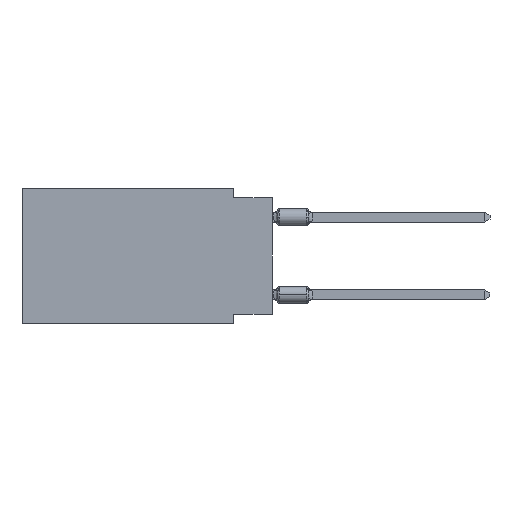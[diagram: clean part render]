
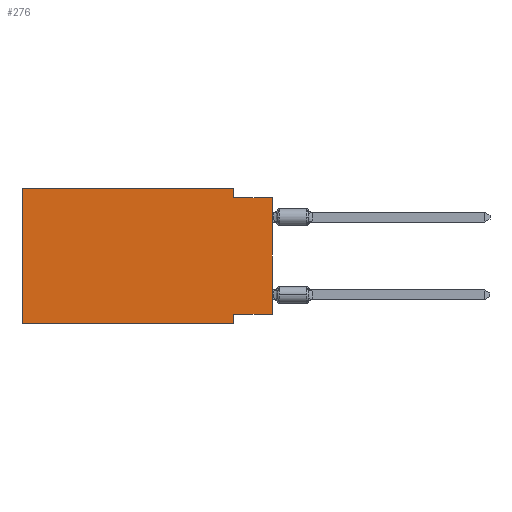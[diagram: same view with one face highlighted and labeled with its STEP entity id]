
A CAD part, left-side view. The second image highlights one B-rep face of the part: STEP entity #276.
In plain terms, the highlighted planar face has unit normal (-1, 0, 0).
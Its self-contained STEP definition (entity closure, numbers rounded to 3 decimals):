
#120 = LINE ( 'NONE', #13959, #4596 ) ;
#276 = ADVANCED_FACE ( 'NONE', ( #6881 ), #6651, .F. ) ;
#680 = DIRECTION ( 'NONE',  ( 0., 0., -1. ) ) ;
#1048 = VERTEX_POINT ( 'NONE', #13488 ) ;
#1146 = CARTESIAN_POINT ( 'NONE',  ( 0., 0., -8.255 ) ) ;
#1196 = VERTEX_POINT ( 'NONE', #15005 ) ;
#1869 = VECTOR ( 'NONE', #13306, 1000. ) ;
#1875 = VERTEX_POINT ( 'NONE', #13358 ) ;
#1990 = VECTOR ( 'NONE', #680, 1000. ) ;
#2413 = VECTOR ( 'NONE', #12455, 1000. ) ;
#2674 = VECTOR ( 'NONE', #12764, 1000. ) ;
#2703 = LINE ( 'NONE', #12063, #1869 ) ;
#2717 = ORIENTED_EDGE ( 'NONE', *, *, #8600, .T. ) ;
#2774 = CARTESIAN_POINT ( 'NONE',  ( 0., 0., 0. ) ) ;
#3293 = LINE ( 'NONE', #3523, #8495 ) ;
#3523 = CARTESIAN_POINT ( 'NONE',  ( 0., 0., -0.635 ) ) ;
#4596 = VECTOR ( 'NONE', #4800, 1000. ) ;
#4697 = CARTESIAN_POINT ( 'NONE',  ( 0., 2.54, -8.255 ) ) ;
#4733 = VECTOR ( 'NONE', #13228, 1000. ) ;
#4800 = DIRECTION ( 'NONE',  ( 0., -1., 0. ) ) ;
#5105 = CARTESIAN_POINT ( 'NONE',  ( 0., 0., -0.635 ) ) ;
#5641 = ORIENTED_EDGE ( 'NONE', *, *, #11929, .F. ) ;
#6446 = VERTEX_POINT ( 'NONE', #13236 ) ;
#6459 = VECTOR ( 'NONE', #9847, 1000. ) ;
#6506 = LINE ( 'NONE', #11202, #1990 ) ;
#6651 = PLANE ( 'NONE',  #11452 ) ;
#6821 = LINE ( 'NONE', #1146, #2674 ) ;
#6881 = FACE_OUTER_BOUND ( 'NONE', #9956, .T. ) ;
#7148 = ORIENTED_EDGE ( 'NONE', *, *, #14521, .F. ) ;
#7232 = CARTESIAN_POINT ( 'NONE',  ( 0., 16.383, -8.89 ) ) ;
#7884 = VERTEX_POINT ( 'NONE', #5105 ) ;
#8495 = VECTOR ( 'NONE', #12664, 1000. ) ;
#8591 = VERTEX_POINT ( 'NONE', #4697 ) ;
#8600 = EDGE_CURVE ( 'NONE', #12624, #7884, #9380, .T. ) ;
#9380 = LINE ( 'NONE', #2774, #4733 ) ;
#9426 = EDGE_CURVE ( 'NONE', #1875, #1048, #10852, .T. ) ;
#9847 = DIRECTION ( 'NONE',  ( 0., -1., 0. ) ) ;
#9956 = EDGE_LOOP ( 'NONE', ( #2717, #11241, #13002, #7148, #12438, #12199, #5641, #10058 ) ) ;
#10058 = ORIENTED_EDGE ( 'NONE', *, *, #12126, .F. ) ;
#10142 = EDGE_CURVE ( 'NONE', #6446, #13594, #6506, .T. ) ;
#10852 = LINE ( 'NONE', #7232, #6459 ) ;
#11202 = CARTESIAN_POINT ( 'NONE',  ( 0., 2.54, 0. ) ) ;
#11241 = ORIENTED_EDGE ( 'NONE', *, *, #13573, .F. ) ;
#11366 = LINE ( 'NONE', #14918, #2413 ) ;
#11452 = AXIS2_PLACEMENT_3D ( 'NONE', #13747, #11579, #13665 ) ;
#11579 = DIRECTION ( 'NONE',  ( 1., 0., 0. ) ) ;
#11929 = EDGE_CURVE ( 'NONE', #8591, #1048, #11366, .T. ) ;
#12063 = CARTESIAN_POINT ( 'NONE',  ( 0., 16.383, 0. ) ) ;
#12126 = EDGE_CURVE ( 'NONE', #12624, #8591, #6821, .T. ) ;
#12199 = ORIENTED_EDGE ( 'NONE', *, *, #9426, .T. ) ;
#12329 = CARTESIAN_POINT ( 'NONE',  ( 0., 0., -8.255 ) ) ;
#12438 = ORIENTED_EDGE ( 'NONE', *, *, #13398, .F. ) ;
#12455 = DIRECTION ( 'NONE',  ( 0., 0., -1. ) ) ;
#12624 = VERTEX_POINT ( 'NONE', #12329 ) ;
#12664 = DIRECTION ( 'NONE',  ( 0., -1., 0. ) ) ;
#12764 = DIRECTION ( 'NONE',  ( 0., 1., 0. ) ) ;
#13002 = ORIENTED_EDGE ( 'NONE', *, *, #10142, .F. ) ;
#13228 = DIRECTION ( 'NONE',  ( 0., 0., 1. ) ) ;
#13236 = CARTESIAN_POINT ( 'NONE',  ( 0., 2.54, 0. ) ) ;
#13306 = DIRECTION ( 'NONE',  ( 0., 0., 1. ) ) ;
#13358 = CARTESIAN_POINT ( 'NONE',  ( 0., 16.383, -8.89 ) ) ;
#13398 = EDGE_CURVE ( 'NONE', #1875, #1196, #2703, .T. ) ;
#13488 = CARTESIAN_POINT ( 'NONE',  ( 0., 2.54, -8.89 ) ) ;
#13573 = EDGE_CURVE ( 'NONE', #13594, #7884, #3293, .T. ) ;
#13594 = VERTEX_POINT ( 'NONE', #14062 ) ;
#13665 = DIRECTION ( 'NONE',  ( 0., 0., -1. ) ) ;
#13747 = CARTESIAN_POINT ( 'NONE',  ( 0., 16.383, 0. ) ) ;
#13959 = CARTESIAN_POINT ( 'NONE',  ( 0., 16.383, 0. ) ) ;
#14062 = CARTESIAN_POINT ( 'NONE',  ( 0., 2.54, -0.635 ) ) ;
#14521 = EDGE_CURVE ( 'NONE', #1196, #6446, #120, .T. ) ;
#14918 = CARTESIAN_POINT ( 'NONE',  ( 0., 2.54, -8.89 ) ) ;
#15005 = CARTESIAN_POINT ( 'NONE',  ( 0., 16.383, 0. ) ) ;
